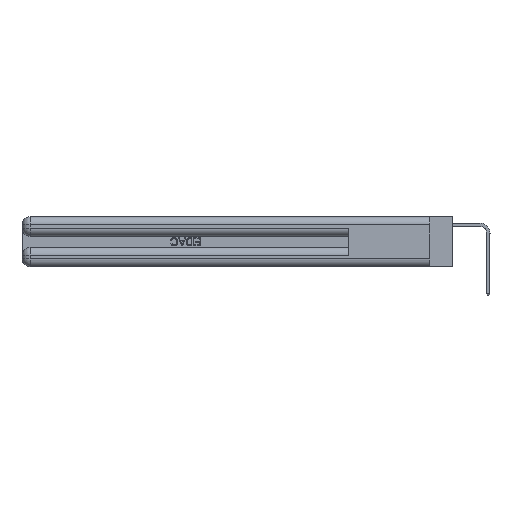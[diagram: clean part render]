
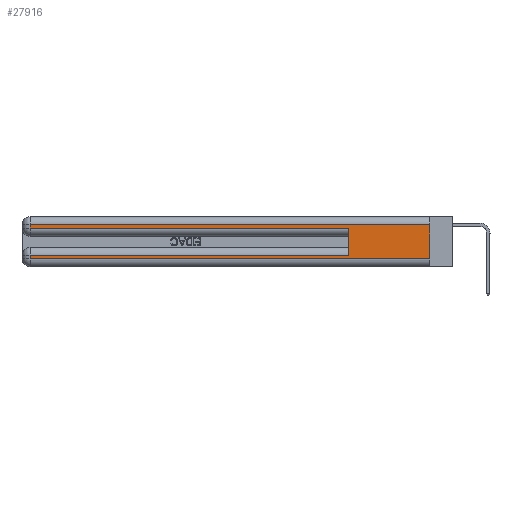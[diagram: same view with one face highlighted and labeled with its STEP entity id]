
A CAD part, left-side view. The second image highlights one B-rep face of the part: STEP entity #27916.
In plain terms, the highlighted planar face has unit normal (-1, 0, 0).
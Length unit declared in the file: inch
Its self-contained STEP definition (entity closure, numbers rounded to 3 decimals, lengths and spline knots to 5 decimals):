
#376 = DIRECTION ( 'NONE',  ( 1., 0., 0. ) ) ;
#951 = CARTESIAN_POINT ( 'NONE',  ( 0., 0.6, 0.285 ) ) ;
#1536 = VERTEX_POINT ( 'NONE', #28301 ) ;
#1805 = DIRECTION ( 'NONE',  ( 0., 1., 0. ) ) ;
#1820 = LINE ( 'NONE', #29073, #26833 ) ;
#3400 = DIRECTION ( 'NONE',  ( 0., 0., -1. ) ) ;
#3855 = VECTOR ( 'NONE', #6804, 39.37008 ) ;
#3923 = CARTESIAN_POINT ( 'NONE',  ( 0., 2.94, 0.085 ) ) ;
#4056 = CARTESIAN_POINT ( 'NONE',  ( 0., 2.94, 0.06 ) ) ;
#4143 = VERTEX_POINT ( 'NONE', #29090 ) ;
#4421 = CARTESIAN_POINT ( 'NONE',  ( 0., 0., 0.31 ) ) ;
#4610 = LINE ( 'NONE', #4421, #3855 ) ;
#5083 = EDGE_CURVE ( 'NONE', #7685, #4143, #7832, .T. ) ;
#5346 = ORIENTED_EDGE ( 'NONE', *, *, #26844, .F. ) ;
#5517 = VERTEX_POINT ( 'NONE', #21018 ) ;
#6374 = ORIENTED_EDGE ( 'NONE', *, *, #14397, .T. ) ;
#6804 = DIRECTION ( 'NONE',  ( 0., 1., 0. ) ) ;
#7414 = CARTESIAN_POINT ( 'NONE',  ( 0., 0., 0.37 ) ) ;
#7585 = VECTOR ( 'NONE', #14341, 39.37008 ) ;
#7685 = VERTEX_POINT ( 'NONE', #4056 ) ;
#7832 = LINE ( 'NONE', #22182, #26517 ) ;
#8074 = CARTESIAN_POINT ( 'NONE',  ( 0., 2.94, 0.37 ) ) ;
#8150 = DIRECTION ( 'NONE',  ( 0., -1., 0. ) ) ;
#8270 = VECTOR ( 'NONE', #18086, 39.37008 ) ;
#9297 = VECTOR ( 'NONE', #3400, 39.37008 ) ;
#9477 = EDGE_CURVE ( 'NONE', #5517, #27129, #13424, .T. ) ;
#10097 = FACE_OUTER_BOUND ( 'NONE', #14478, .T. ) ;
#10106 = EDGE_CURVE ( 'NONE', #5517, #16331, #26971, .T. ) ;
#10559 = EDGE_CURVE ( 'NONE', #22497, #1536, #15509, .T. ) ;
#11525 = ORIENTED_EDGE ( 'NONE', *, *, #10559, .T. ) ;
#12353 = ORIENTED_EDGE ( 'NONE', *, *, #29865, .T. ) ;
#12467 = CARTESIAN_POINT ( 'NONE',  ( 0., 2.94, 0.31 ) ) ;
#13424 = LINE ( 'NONE', #15902, #19666 ) ;
#14341 = DIRECTION ( 'NONE',  ( 0., 0., -1. ) ) ;
#14397 = EDGE_CURVE ( 'NONE', #18287, #22497, #4610, .T. ) ;
#14478 = EDGE_LOOP ( 'NONE', ( #5346, #6374, #11525, #12353, #30357, #26603, #21856, #22898 ) ) ;
#14480 = PLANE ( 'NONE',  #20760 ) ;
#15509 = LINE ( 'NONE', #8074, #9297 ) ;
#15771 = CARTESIAN_POINT ( 'NONE',  ( 0., 0.6, 0.145 ) ) ;
#15902 = CARTESIAN_POINT ( 'NONE',  ( 0., 0., 0.085 ) ) ;
#16331 = VERTEX_POINT ( 'NONE', #951 ) ;
#16818 = DIRECTION ( 'NONE',  ( 0., 0., -1. ) ) ;
#17333 = DIRECTION ( 'NONE',  ( 0., -1., 0. ) ) ;
#17621 = CARTESIAN_POINT ( 'NONE',  ( 0., 2.94, 0.37 ) ) ;
#17652 = EDGE_CURVE ( 'NONE', #27129, #7685, #23406, .T. ) ;
#17986 = CARTESIAN_POINT ( 'NONE',  ( 0., 0., 0.31 ) ) ;
#18086 = DIRECTION ( 'NONE',  ( 0., 0., 1. ) ) ;
#18287 = VERTEX_POINT ( 'NONE', #17986 ) ;
#19666 = VECTOR ( 'NONE', #1805, 39.37008 ) ;
#20018 = LINE ( 'NONE', #26013, #7585 ) ;
#20760 = AXIS2_PLACEMENT_3D ( 'NONE', #7414, #376, #16818 ) ;
#21018 = CARTESIAN_POINT ( 'NONE',  ( 0., 0.6, 0.085 ) ) ;
#21856 = ORIENTED_EDGE ( 'NONE', *, *, #17652, .T. ) ;
#22182 = CARTESIAN_POINT ( 'NONE',  ( 0., 0., 0.06 ) ) ;
#22497 = VERTEX_POINT ( 'NONE', #12467 ) ;
#22898 = ORIENTED_EDGE ( 'NONE', *, *, #5083, .T. ) ;
#23406 = LINE ( 'NONE', #17621, #28941 ) ;
#26013 = CARTESIAN_POINT ( 'NONE',  ( 0., 0., 0.37 ) ) ;
#26517 = VECTOR ( 'NONE', #8150, 39.37008 ) ;
#26603 = ORIENTED_EDGE ( 'NONE', *, *, #9477, .T. ) ;
#26833 = VECTOR ( 'NONE', #17333, 39.37008 ) ;
#26844 = EDGE_CURVE ( 'NONE', #18287, #4143, #20018, .T. ) ;
#26971 = LINE ( 'NONE', #15771, #8270 ) ;
#27129 = VERTEX_POINT ( 'NONE', #3923 ) ;
#27916 = ADVANCED_FACE ( 'NONE', ( #10097 ), #14480, .F. ) ;
#28301 = CARTESIAN_POINT ( 'NONE',  ( 0., 2.94, 0.285 ) ) ;
#28941 = VECTOR ( 'NONE', #29367, 39.37008 ) ;
#29073 = CARTESIAN_POINT ( 'NONE',  ( 0., 0., 0.285 ) ) ;
#29090 = CARTESIAN_POINT ( 'NONE',  ( 0., 0., 0.06 ) ) ;
#29367 = DIRECTION ( 'NONE',  ( 0., 0., -1. ) ) ;
#29865 = EDGE_CURVE ( 'NONE', #1536, #16331, #1820, .T. ) ;
#30357 = ORIENTED_EDGE ( 'NONE', *, *, #10106, .F. ) ;
